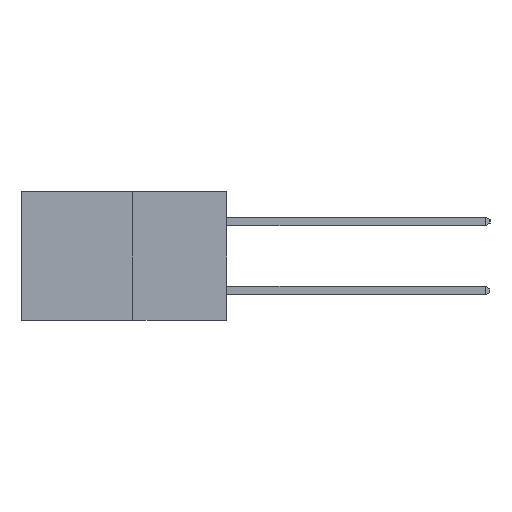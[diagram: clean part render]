
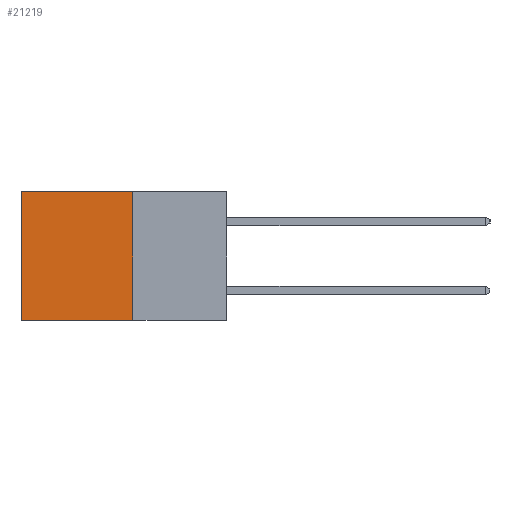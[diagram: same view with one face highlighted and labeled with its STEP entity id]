
A CAD part, left-side view. The second image highlights one B-rep face of the part: STEP entity #21219.
In plain terms, the highlighted planar face has unit normal (-1, 0, 0).
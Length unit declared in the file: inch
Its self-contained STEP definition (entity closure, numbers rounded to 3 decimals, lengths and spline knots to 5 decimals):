
#1620 = VERTEX_POINT ( 'NONE', #8467 ) ;
#1851 = VECTOR ( 'NONE', #7471, 39.37008 ) ;
#4157 = CARTESIAN_POINT ( 'NONE',  ( 0.277, 0.27, 0. ) ) ;
#4681 = CARTESIAN_POINT ( 'NONE',  ( 0.277, 0.27, -0.37 ) ) ;
#4702 = DIRECTION ( 'NONE',  ( 0., 0., -1. ) ) ;
#5282 = VECTOR ( 'NONE', #9285, 39.37008 ) ;
#6235 = VERTEX_POINT ( 'NONE', #4157 ) ;
#7031 = LINE ( 'NONE', #24494, #1851 ) ;
#7220 = VERTEX_POINT ( 'NONE', #21443 ) ;
#7471 = DIRECTION ( 'NONE',  ( 0., 1., 0. ) ) ;
#8467 = CARTESIAN_POINT ( 'NONE',  ( 0.277, 0.27, -0.37 ) ) ;
#9285 = DIRECTION ( 'NONE',  ( 0., 1., 0. ) ) ;
#9563 = FACE_OUTER_BOUND ( 'NONE', #9592, .T. ) ;
#9592 = EDGE_LOOP ( 'NONE', ( #23922, #23852, #22255, #20217 ) ) ;
#9656 = EDGE_CURVE ( 'NONE', #1620, #14099, #7031, .T. ) ;
#10488 = DIRECTION ( 'NONE',  ( 1., 0., 0. ) ) ;
#14099 = VERTEX_POINT ( 'NONE', #16763 ) ;
#14257 = CARTESIAN_POINT ( 'NONE',  ( 0.277, 0.27, -0.37 ) ) ;
#14845 = EDGE_CURVE ( 'NONE', #6235, #7220, #15490, .T. ) ;
#15490 = LINE ( 'NONE', #22575, #5282 ) ;
#15853 = EDGE_CURVE ( 'NONE', #6235, #1620, #18684, .T. ) ;
#16763 = CARTESIAN_POINT ( 'NONE',  ( 0.277, 0.59, -0.37 ) ) ;
#17526 = VECTOR ( 'NONE', #4702, 39.37008 ) ;
#18272 = DIRECTION ( 'NONE',  ( 0., 0., -1. ) ) ;
#18684 = LINE ( 'NONE', #14257, #17526 ) ;
#19173 = EDGE_CURVE ( 'NONE', #7220, #14099, #21270, .T. ) ;
#20095 = VECTOR ( 'NONE', #18272, 39.37008 ) ;
#20164 = CARTESIAN_POINT ( 'NONE',  ( 0.277, 0.59, -0.37 ) ) ;
#20217 = ORIENTED_EDGE ( 'NONE', *, *, #14845, .T. ) ;
#20271 = AXIS2_PLACEMENT_3D ( 'NONE', #4681, #10488, #23772 ) ;
#21219 = ADVANCED_FACE ( 'NONE', ( #9563 ), #21869, .F. ) ;
#21270 = LINE ( 'NONE', #20164, #20095 ) ;
#21443 = CARTESIAN_POINT ( 'NONE',  ( 0.277, 0.59, 0. ) ) ;
#21869 = PLANE ( 'NONE',  #20271 ) ;
#22255 = ORIENTED_EDGE ( 'NONE', *, *, #15853, .F. ) ;
#22575 = CARTESIAN_POINT ( 'NONE',  ( 0.277, 0.27, 0. ) ) ;
#23772 = DIRECTION ( 'NONE',  ( 0., 0., -1. ) ) ;
#23852 = ORIENTED_EDGE ( 'NONE', *, *, #9656, .F. ) ;
#23922 = ORIENTED_EDGE ( 'NONE', *, *, #19173, .T. ) ;
#24494 = CARTESIAN_POINT ( 'NONE',  ( 0.277, 0.27, -0.37 ) ) ;
